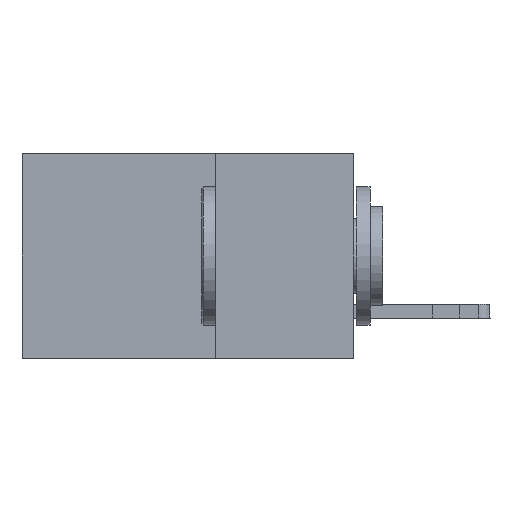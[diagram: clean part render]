
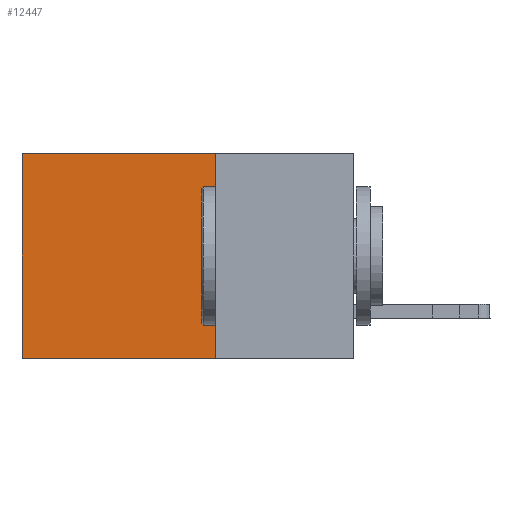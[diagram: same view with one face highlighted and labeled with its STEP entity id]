
A CAD part, left-side view. The second image highlights one B-rep face of the part: STEP entity #12447.
In plain terms, the highlighted planar face has unit normal (-1, 0, 0).
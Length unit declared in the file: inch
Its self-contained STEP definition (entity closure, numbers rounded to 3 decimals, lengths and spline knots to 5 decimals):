
#391 = DIRECTION ( 'NONE',  ( 0., 1., 0. ) ) ;
#501 = PLANE ( 'NONE',  #8901 ) ;
#594 = VERTEX_POINT ( 'NONE', #14729 ) ;
#1396 = LINE ( 'NONE', #14321, #2011 ) ;
#2011 = VECTOR ( 'NONE', #13793, 39.37008 ) ;
#2400 = LINE ( 'NONE', #12775, #22720 ) ;
#2655 = DIRECTION ( 'NONE',  ( 1., 0., 0. ) ) ;
#3207 = EDGE_CURVE ( 'NONE', #10574, #9443, #23259, .T. ) ;
#3687 = EDGE_CURVE ( 'NONE', #9443, #594, #14754, .T. ) ;
#6886 = CARTESIAN_POINT ( 'NONE',  ( 0.2875, 0.25, -0.37 ) ) ;
#7331 = ORIENTED_EDGE ( 'NONE', *, *, #15908, .F. ) ;
#8901 = AXIS2_PLACEMENT_3D ( 'NONE', #14667, #2655, #10628 ) ;
#9443 = VERTEX_POINT ( 'NONE', #24723 ) ;
#10550 = ORIENTED_EDGE ( 'NONE', *, *, #3207, .T. ) ;
#10574 = VERTEX_POINT ( 'NONE', #15621 ) ;
#10628 = DIRECTION ( 'NONE',  ( 0., 0., -1. ) ) ;
#11737 = ORIENTED_EDGE ( 'NONE', *, *, #24106, .F. ) ;
#12376 = VECTOR ( 'NONE', #13000, 39.37008 ) ;
#12447 = ADVANCED_FACE ( 'NONE', ( #19381 ), #501, .F. ) ;
#12775 = CARTESIAN_POINT ( 'NONE',  ( 0.2875, 0.25, -0.37 ) ) ;
#13000 = DIRECTION ( 'NONE',  ( 0., 1., 0. ) ) ;
#13793 = DIRECTION ( 'NONE',  ( 0., 0., -1. ) ) ;
#14321 = CARTESIAN_POINT ( 'NONE',  ( 0.2875, 0.25, 0. ) ) ;
#14344 = CARTESIAN_POINT ( 'NONE',  ( 0.2875, 0.6, 0. ) ) ;
#14667 = CARTESIAN_POINT ( 'NONE',  ( 0.2875, 0.25, 0. ) ) ;
#14729 = CARTESIAN_POINT ( 'NONE',  ( 0.2875, 0.6, -0.37 ) ) ;
#14754 = LINE ( 'NONE', #14344, #18436 ) ;
#15621 = CARTESIAN_POINT ( 'NONE',  ( 0.2875, 0.25, 0. ) ) ;
#15908 = EDGE_CURVE ( 'NONE', #26079, #594, #2400, .T. ) ;
#18436 = VECTOR ( 'NONE', #18676, 39.37008 ) ;
#18676 = DIRECTION ( 'NONE',  ( 0., 0., -1. ) ) ;
#19081 = CARTESIAN_POINT ( 'NONE',  ( 0.2875, 0.25, 0. ) ) ;
#19381 = FACE_OUTER_BOUND ( 'NONE', #26191, .T. ) ;
#22720 = VECTOR ( 'NONE', #391, 39.37008 ) ;
#23259 = LINE ( 'NONE', #19081, #12376 ) ;
#23351 = ORIENTED_EDGE ( 'NONE', *, *, #3687, .T. ) ;
#24106 = EDGE_CURVE ( 'NONE', #10574, #26079, #1396, .T. ) ;
#24723 = CARTESIAN_POINT ( 'NONE',  ( 0.2875, 0.6, 0. ) ) ;
#26079 = VERTEX_POINT ( 'NONE', #6886 ) ;
#26191 = EDGE_LOOP ( 'NONE', ( #23351, #7331, #11737, #10550 ) ) ;
